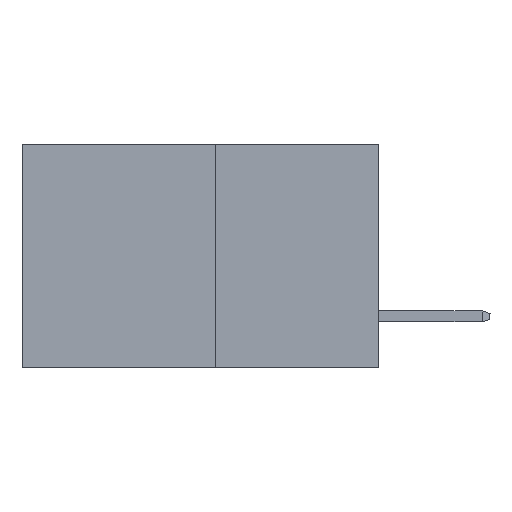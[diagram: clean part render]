
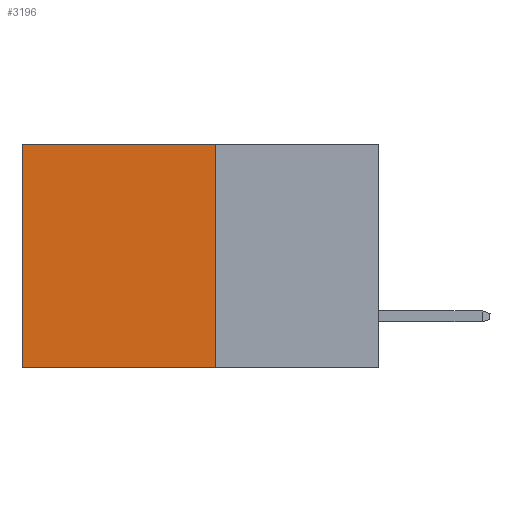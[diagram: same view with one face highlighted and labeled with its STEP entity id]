
A CAD part, left-side view. The second image highlights one B-rep face of the part: STEP entity #3196.
In plain terms, the highlighted planar face has unit normal (-1, 0, 0).
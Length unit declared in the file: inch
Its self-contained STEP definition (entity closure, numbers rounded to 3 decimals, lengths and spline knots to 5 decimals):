
#94 = VECTOR ( 'NONE', #7840, 39.37008 ) ;
#1062 = CARTESIAN_POINT ( 'NONE',  ( 0.277, 0.27, -0.37 ) ) ;
#3196 = ADVANCED_FACE ( 'NONE', ( #3427 ), #3962, .F. ) ;
#3427 = FACE_OUTER_BOUND ( 'NONE', #5007, .T. ) ;
#3548 = ORIENTED_EDGE ( 'NONE', *, *, #7697, .F. ) ;
#3550 = DIRECTION ( 'NONE',  ( 0., 0., -1. ) ) ;
#3602 = DIRECTION ( 'NONE',  ( 1., 0., 0. ) ) ;
#3784 = CARTESIAN_POINT ( 'NONE',  ( 0.277, 0.27, -0.37 ) ) ;
#3962 = PLANE ( 'NONE',  #4138 ) ;
#4138 = AXIS2_PLACEMENT_3D ( 'NONE', #3784, #3602, #3550 ) ;
#5007 = EDGE_LOOP ( 'NONE', ( #16563, #3548, #20786, #18073 ) ) ;
#5504 = DIRECTION ( 'NONE',  ( 0., 0., -1. ) ) ;
#5679 = CARTESIAN_POINT ( 'NONE',  ( 0.277, 0.59, -0.37 ) ) ;
#7077 = LINE ( 'NONE', #9199, #19326 ) ;
#7232 = VERTEX_POINT ( 'NONE', #12272 ) ;
#7640 = CARTESIAN_POINT ( 'NONE',  ( 0.277, 0.27, -0.37 ) ) ;
#7697 = EDGE_CURVE ( 'NONE', #7232, #21488, #13946, .T. ) ;
#7840 = DIRECTION ( 'NONE',  ( 0., 1., 0. ) ) ;
#7922 = EDGE_CURVE ( 'NONE', #15037, #21488, #21391, .T. ) ;
#8685 = VECTOR ( 'NONE', #5504, 39.37008 ) ;
#9049 = CARTESIAN_POINT ( 'NONE',  ( 0.277, 0.27, 0. ) ) ;
#9199 = CARTESIAN_POINT ( 'NONE',  ( 0.277, 0.27, 0. ) ) ;
#10869 = VECTOR ( 'NONE', #11031, 39.37008 ) ;
#10875 = DIRECTION ( 'NONE',  ( 0., 1., 0. ) ) ;
#11031 = DIRECTION ( 'NONE',  ( 0., 0., -1. ) ) ;
#12272 = CARTESIAN_POINT ( 'NONE',  ( 0.277, 0.27, -0.37 ) ) ;
#12393 = EDGE_CURVE ( 'NONE', #12942, #7232, #18748, .T. ) ;
#12942 = VERTEX_POINT ( 'NONE', #9049 ) ;
#13865 = CARTESIAN_POINT ( 'NONE',  ( 0.277, 0.59, -0.37 ) ) ;
#13946 = LINE ( 'NONE', #7640, #94 ) ;
#14706 = CARTESIAN_POINT ( 'NONE',  ( 0.277, 0.59, 0. ) ) ;
#15037 = VERTEX_POINT ( 'NONE', #14706 ) ;
#16563 = ORIENTED_EDGE ( 'NONE', *, *, #7922, .T. ) ;
#16675 = EDGE_CURVE ( 'NONE', #12942, #15037, #7077, .T. ) ;
#18073 = ORIENTED_EDGE ( 'NONE', *, *, #16675, .T. ) ;
#18748 = LINE ( 'NONE', #1062, #10869 ) ;
#19326 = VECTOR ( 'NONE', #10875, 39.37008 ) ;
#20786 = ORIENTED_EDGE ( 'NONE', *, *, #12393, .F. ) ;
#21391 = LINE ( 'NONE', #5679, #8685 ) ;
#21488 = VERTEX_POINT ( 'NONE', #13865 ) ;
